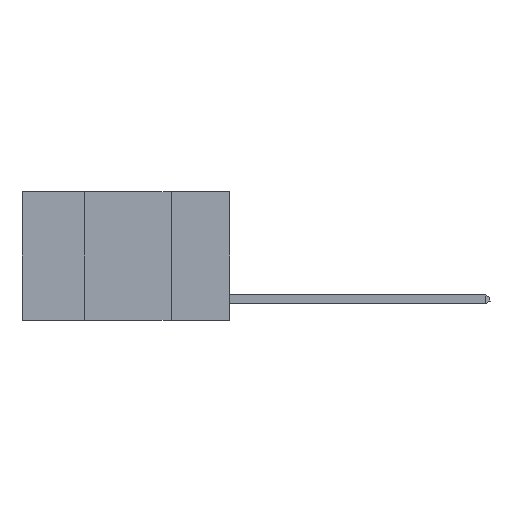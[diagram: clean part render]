
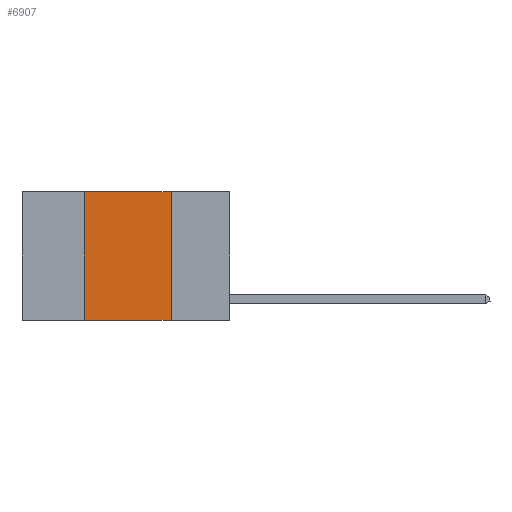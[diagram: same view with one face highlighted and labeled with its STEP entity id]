
A CAD part, left-side view. The second image highlights one B-rep face of the part: STEP entity #6907.
In plain terms, the highlighted planar face has unit normal (-1, 0, 0).
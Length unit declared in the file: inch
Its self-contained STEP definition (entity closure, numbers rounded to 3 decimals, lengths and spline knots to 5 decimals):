
#104 = PLANE ( 'NONE',  #12025 ) ;
#402 = ORIENTED_EDGE ( 'NONE', *, *, #1997, .F. ) ;
#635 = EDGE_CURVE ( 'NONE', #5415, #1895, #15201, .T. ) ;
#1895 = VERTEX_POINT ( 'NONE', #4945 ) ;
#1997 = EDGE_CURVE ( 'NONE', #7254, #5415, #5211, .T. ) ;
#2434 = CARTESIAN_POINT ( 'NONE',  ( 0., 0.6, -0.37 ) ) ;
#2529 = DIRECTION ( 'NONE',  ( 0., 0., 1. ) ) ;
#3391 = LINE ( 'NONE', #7428, #8161 ) ;
#3662 = DIRECTION ( 'NONE',  ( 0., -1., 0. ) ) ;
#3920 = CARTESIAN_POINT ( 'NONE',  ( 0., 0.42, 0. ) ) ;
#4204 = DIRECTION ( 'NONE',  ( 1., 0., 0. ) ) ;
#4760 = LINE ( 'NONE', #2434, #13618 ) ;
#4945 = CARTESIAN_POINT ( 'NONE',  ( 0., 0.17, 0. ) ) ;
#5022 = DIRECTION ( 'NONE',  ( 0., -1., 0. ) ) ;
#5211 = LINE ( 'NONE', #16393, #13349 ) ;
#5415 = VERTEX_POINT ( 'NONE', #3920 ) ;
#5579 = CARTESIAN_POINT ( 'NONE',  ( 0., 0.6, 0. ) ) ;
#6907 = ADVANCED_FACE ( 'NONE', ( #12345 ), #104, .F. ) ;
#7254 = VERTEX_POINT ( 'NONE', #16641 ) ;
#7428 = CARTESIAN_POINT ( 'NONE',  ( 0., 0.17, 0. ) ) ;
#7613 = VECTOR ( 'NONE', #3662, 39.37008 ) ;
#8161 = VECTOR ( 'NONE', #14196, 39.37008 ) ;
#8402 = CARTESIAN_POINT ( 'NONE',  ( 0., 0.6, 0. ) ) ;
#8856 = VERTEX_POINT ( 'NONE', #13313 ) ;
#9089 = ORIENTED_EDGE ( 'NONE', *, *, #15940, .F. ) ;
#9162 = ORIENTED_EDGE ( 'NONE', *, *, #16868, .T. ) ;
#9662 = DIRECTION ( 'NONE',  ( 0., 0., -1. ) ) ;
#11402 = EDGE_LOOP ( 'NONE', ( #9089, #14788, #402, #9162 ) ) ;
#12025 = AXIS2_PLACEMENT_3D ( 'NONE', #5579, #4204, #9662 ) ;
#12345 = FACE_OUTER_BOUND ( 'NONE', #11402, .T. ) ;
#13313 = CARTESIAN_POINT ( 'NONE',  ( 0., 0.17, -0.37 ) ) ;
#13349 = VECTOR ( 'NONE', #2529, 39.37008 ) ;
#13618 = VECTOR ( 'NONE', #5022, 39.37008 ) ;
#14196 = DIRECTION ( 'NONE',  ( 0., 0., -1. ) ) ;
#14788 = ORIENTED_EDGE ( 'NONE', *, *, #635, .F. ) ;
#15201 = LINE ( 'NONE', #8402, #7613 ) ;
#15940 = EDGE_CURVE ( 'NONE', #1895, #8856, #3391, .T. ) ;
#16393 = CARTESIAN_POINT ( 'NONE',  ( 0., 0.42, 0. ) ) ;
#16641 = CARTESIAN_POINT ( 'NONE',  ( 0., 0.42, -0.37 ) ) ;
#16868 = EDGE_CURVE ( 'NONE', #7254, #8856, #4760, .T. ) ;
